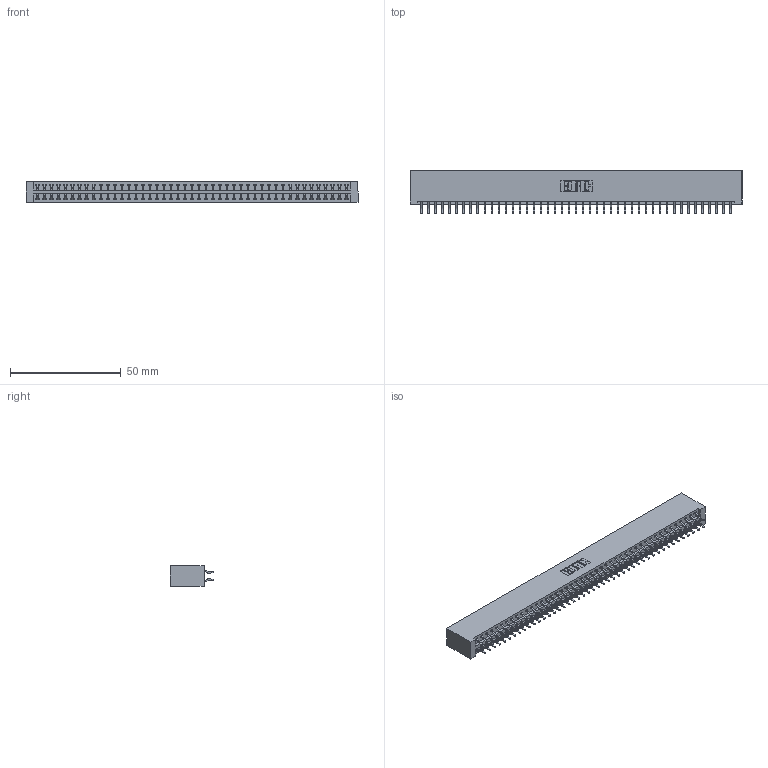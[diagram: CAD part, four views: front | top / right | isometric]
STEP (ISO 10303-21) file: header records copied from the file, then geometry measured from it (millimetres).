
FILE_DESCRIPTION (( 'STEP AP203' ), '1' );
FILE_NAME ('396-090-556-201.STEP', '2019-10-31T02:10:36', ( '' ), ( '' ), 'SwSTEP 2.0', 'SolidWorks 2016', '' );
FILE_SCHEMA (( 'CONFIG_CONTROL_DESIGN' ));
Length unit declared in the file: inch
Products named in the file (3): 396-090-556-201; 345-292-001_556 Tail; 346 Part_No Mounting Lugs
Assembly tree (91 placements, depth 2):
  396-090-556-201
    346 Part_No Mounting Lugs
    345-292-001_556 Tail  x90
Bounding box: 150.11 x 19.57 x 9.4 mm (x, y, z)
Volume: 15231 mm3; surface area: 21062.8 mm2
Topology: 91 solids, 91 shells, 5334 faces, 15875 edges, 10462 vertices
Faces by surface type: plane 3582, cylinder 1752
Entity records: 28907 total; most frequent: CARTESIAN_POINT 4772, ORIENTED_EDGE 4694, DIRECTION 4239, EDGE_CURVE 2347, LINE 2035, VECTOR 2035, VERTEX_POINT 1562, AXIS2_PLACEMENT_3D 1102
